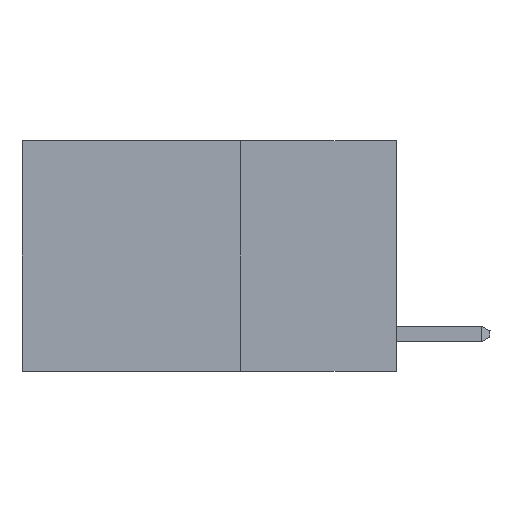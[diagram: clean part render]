
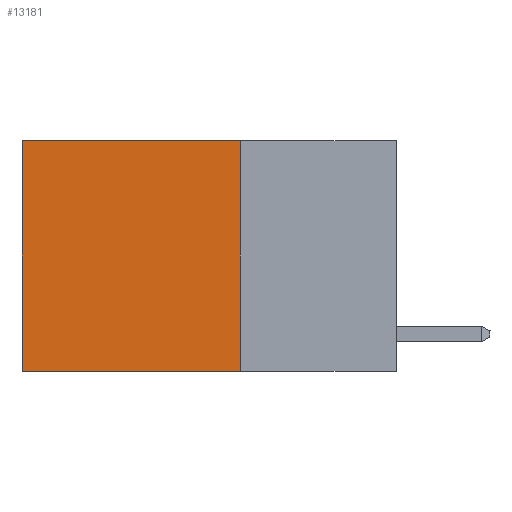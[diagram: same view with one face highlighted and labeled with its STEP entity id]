
A CAD part, left-side view. The second image highlights one B-rep face of the part: STEP entity #13181.
In plain terms, the highlighted planar face has unit normal (-1, 0, 0).
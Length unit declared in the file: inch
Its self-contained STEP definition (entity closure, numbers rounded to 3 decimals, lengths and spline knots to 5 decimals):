
#68 = DIRECTION ( 'NONE',  ( 1., 0., 0. ) ) ;
#377 = LINE ( 'NONE', #2238, #3125 ) ;
#571 = ORIENTED_EDGE ( 'NONE', *, *, #7825, .F. ) ;
#763 = ORIENTED_EDGE ( 'NONE', *, *, #2784, .T. ) ;
#1278 = CARTESIAN_POINT ( 'NONE',  ( 0.2625, 0.25, 0. ) ) ;
#2238 = CARTESIAN_POINT ( 'NONE',  ( 0.2625, 0.25, 0. ) ) ;
#2784 = EDGE_CURVE ( 'NONE', #7315, #12004, #7126, .T. ) ;
#2892 = CARTESIAN_POINT ( 'NONE',  ( 0.2625, 0.25, 0. ) ) ;
#3090 = EDGE_CURVE ( 'NONE', #12004, #9358, #6196, .T. ) ;
#3125 = VECTOR ( 'NONE', #11634, 39.37008 ) ;
#3705 = CARTESIAN_POINT ( 'NONE',  ( 0.2625, 0.6, 0. ) ) ;
#4753 = PLANE ( 'NONE',  #7828 ) ;
#5262 = EDGE_LOOP ( 'NONE', ( #10631, #571, #10209, #763 ) ) ;
#5784 = CARTESIAN_POINT ( 'NONE',  ( 0.2625, 0.6, -0.37 ) ) ;
#5933 = CARTESIAN_POINT ( 'NONE',  ( 0.2625, 0.25, 0. ) ) ;
#6032 = VECTOR ( 'NONE', #15062, 39.37008 ) ;
#6196 = LINE ( 'NONE', #13914, #6032 ) ;
#6387 = VERTEX_POINT ( 'NONE', #14567 ) ;
#7044 = VECTOR ( 'NONE', #15025, 39.37008 ) ;
#7126 = LINE ( 'NONE', #2892, #13317 ) ;
#7315 = VERTEX_POINT ( 'NONE', #1278 ) ;
#7413 = LINE ( 'NONE', #8116, #7044 ) ;
#7825 = EDGE_CURVE ( 'NONE', #6387, #9358, #7413, .T. ) ;
#7828 = AXIS2_PLACEMENT_3D ( 'NONE', #5933, #68, #8327 ) ;
#8116 = CARTESIAN_POINT ( 'NONE',  ( 0.2625, 0.25, -0.37 ) ) ;
#8327 = DIRECTION ( 'NONE',  ( 0., 0., -1. ) ) ;
#9173 = EDGE_CURVE ( 'NONE', #7315, #6387, #377, .T. ) ;
#9358 = VERTEX_POINT ( 'NONE', #5784 ) ;
#9955 = DIRECTION ( 'NONE',  ( 0., 1., 0. ) ) ;
#10201 = FACE_OUTER_BOUND ( 'NONE', #5262, .T. ) ;
#10209 = ORIENTED_EDGE ( 'NONE', *, *, #9173, .F. ) ;
#10631 = ORIENTED_EDGE ( 'NONE', *, *, #3090, .T. ) ;
#11634 = DIRECTION ( 'NONE',  ( 0., 0., -1. ) ) ;
#12004 = VERTEX_POINT ( 'NONE', #3705 ) ;
#13181 = ADVANCED_FACE ( 'NONE', ( #10201 ), #4753, .F. ) ;
#13317 = VECTOR ( 'NONE', #9955, 39.37008 ) ;
#13914 = CARTESIAN_POINT ( 'NONE',  ( 0.2625, 0.6, 0. ) ) ;
#14567 = CARTESIAN_POINT ( 'NONE',  ( 0.2625, 0.25, -0.37 ) ) ;
#15025 = DIRECTION ( 'NONE',  ( 0., 1., 0. ) ) ;
#15062 = DIRECTION ( 'NONE',  ( 0., 0., -1. ) ) ;
